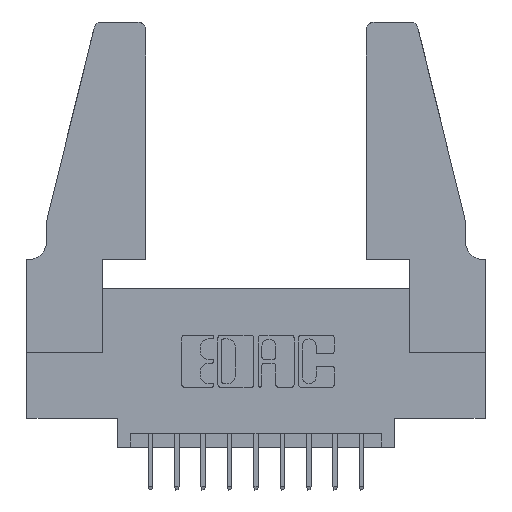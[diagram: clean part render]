
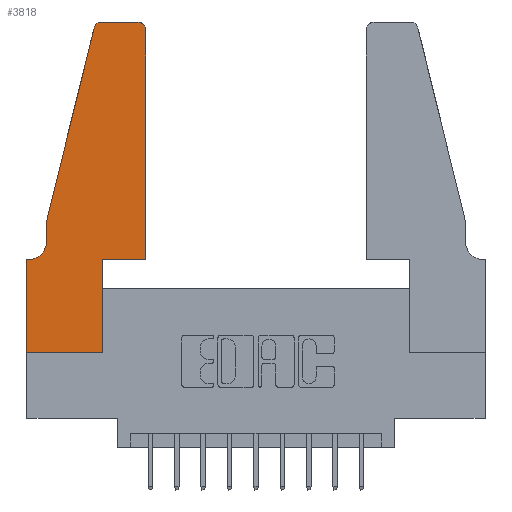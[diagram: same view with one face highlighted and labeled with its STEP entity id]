
A CAD part, top view. The second image highlights one B-rep face of the part: STEP entity #3818.
In plain terms, the highlighted planar face has unit normal (0, 0, 1).
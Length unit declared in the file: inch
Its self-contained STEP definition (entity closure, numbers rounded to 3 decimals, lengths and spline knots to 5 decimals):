
#101 = AXIS2_PLACEMENT_3D ( 'NONE', #13652, #8161, #7247 ) ;
#173 = CIRCLE ( 'NONE', #12254, 0.03 ) ;
#310 = CARTESIAN_POINT ( 'NONE',  ( 0.25487, 1.22718, 0.37 ) ) ;
#331 = DIRECTION ( 'NONE',  ( 0., 0., -1. ) ) ;
#516 = VECTOR ( 'NONE', #9417, 39.37008 ) ;
#571 = ORIENTED_EDGE ( 'NONE', *, *, #11517, .T. ) ;
#584 = DIRECTION ( 'NONE',  ( -0.239, -0.971, 0. ) ) ;
#972 = CARTESIAN_POINT ( 'NONE',  ( 0., 0., 0.37 ) ) ;
#1121 = LINE ( 'NONE', #11549, #13678 ) ;
#1203 = DIRECTION ( 'NONE',  ( 0., 0., 1. ) ) ;
#1227 = CARTESIAN_POINT ( 'NONE',  ( 0.2865, 0.35, 0.37 ) ) ;
#1270 = VERTEX_POINT ( 'NONE', #7177 ) ;
#1333 = ORIENTED_EDGE ( 'NONE', *, *, #12567, .T. ) ;
#2077 = CARTESIAN_POINT ( 'NONE',  ( 0.4505, 0.35, 0.37 ) ) ;
#2159 = ORIENTED_EDGE ( 'NONE', *, *, #5766, .T. ) ;
#2415 = VECTOR ( 'NONE', #11024, 39.37008 ) ;
#3048 = VERTEX_POINT ( 'NONE', #10202 ) ;
#3243 = CARTESIAN_POINT ( 'NONE',  ( 0.284, 1.25, 0.37 ) ) ;
#3503 = LINE ( 'NONE', #972, #10689 ) ;
#3506 = CARTESIAN_POINT ( 'NONE',  ( 0.0755, 0.42, 0.37 ) ) ;
#3565 = DIRECTION ( 'NONE',  ( -1., 0., 0. ) ) ;
#3571 = EDGE_LOOP ( 'NONE', ( #6645, #12556, #571, #2159, #7441, #1333, #13714, #7358, #8673, #13281, #11653, #7525 ) ) ;
#3768 = VERTEX_POINT ( 'NONE', #8648 ) ;
#3787 = VECTOR ( 'NONE', #7420, 39.37008 ) ;
#3810 = VECTOR ( 'NONE', #8436, 39.37008 ) ;
#3818 = ADVANCED_FACE ( 'NONE', ( #10408 ), #4012, .T. ) ;
#4012 = PLANE ( 'NONE',  #101 ) ;
#4269 = CARTESIAN_POINT ( 'NONE',  ( 0.4505, 0.35, 0.37 ) ) ;
#4739 = DIRECTION ( 'NONE',  ( 1., 0., 0. ) ) ;
#5197 = DIRECTION ( 'NONE',  ( 0., 1., 0. ) ) ;
#5241 = VERTEX_POINT ( 'NONE', #3243 ) ;
#5455 = CARTESIAN_POINT ( 'NONE',  ( 0.4505, 1.22, 0.37 ) ) ;
#5630 = CIRCLE ( 'NONE', #12448, 0.03 ) ;
#5703 = CARTESIAN_POINT ( 'NONE',  ( 0.284, 1.22, 0.37 ) ) ;
#5766 = EDGE_CURVE ( 'NONE', #6550, #9690, #7827, .T. ) ;
#5801 = CARTESIAN_POINT ( 'NONE',  ( 0.0755, 0.35, 0.37 ) ) ;
#5875 = VERTEX_POINT ( 'NONE', #4269 ) ;
#6411 = DIRECTION ( 'NONE',  ( 0., -1., 0. ) ) ;
#6478 = EDGE_CURVE ( 'NONE', #8548, #5875, #11326, .T. ) ;
#6481 = EDGE_CURVE ( 'NONE', #3048, #9802, #1121, .T. ) ;
#6500 = EDGE_CURVE ( 'NONE', #1270, #5241, #12181, .T. ) ;
#6550 = VERTEX_POINT ( 'NONE', #7520 ) ;
#6645 = ORIENTED_EDGE ( 'NONE', *, *, #6500, .T. ) ;
#7027 = EDGE_CURVE ( 'NONE', #9690, #3768, #12182, .T. ) ;
#7177 = CARTESIAN_POINT ( 'NONE',  ( 0.4205, 1.25, 0.37 ) ) ;
#7247 = DIRECTION ( 'NONE',  ( 1., 0., 0. ) ) ;
#7358 = ORIENTED_EDGE ( 'NONE', *, *, #9255, .T. ) ;
#7384 = LINE ( 'NONE', #11530, #516 ) ;
#7394 = CARTESIAN_POINT ( 'NONE',  ( 0.0755, 0.5, 0.37 ) ) ;
#7420 = DIRECTION ( 'NONE',  ( -1., 0., 0. ) ) ;
#7441 = ORIENTED_EDGE ( 'NONE', *, *, #7027, .T. ) ;
#7478 = VERTEX_POINT ( 'NONE', #9948 ) ;
#7520 = CARTESIAN_POINT ( 'NONE',  ( 0.0755, 0.5, 0.37 ) ) ;
#7525 = ORIENTED_EDGE ( 'NONE', *, *, #7656, .T. ) ;
#7656 = EDGE_CURVE ( 'NONE', #13601, #1270, #173, .T. ) ;
#7827 = LINE ( 'NONE', #7394, #3810 ) ;
#7829 = EDGE_CURVE ( 'NONE', #7478, #8548, #12726, .T. ) ;
#8161 = DIRECTION ( 'NONE',  ( 0., 0., 1. ) ) ;
#8436 = DIRECTION ( 'NONE',  ( 0., -1., 0. ) ) ;
#8548 = VERTEX_POINT ( 'NONE', #1227 ) ;
#8566 = CARTESIAN_POINT ( 'NONE',  ( 0.2605, 1.25, 0.37 ) ) ;
#8606 = LINE ( 'NONE', #5801, #2415 ) ;
#8629 = LINE ( 'NONE', #12074, #9614 ) ;
#8648 = CARTESIAN_POINT ( 'NONE',  ( 0.0055, 0.35, 0.37 ) ) ;
#8673 = ORIENTED_EDGE ( 'NONE', *, *, #7829, .T. ) ;
#8932 = CARTESIAN_POINT ( 'NONE',  ( 0.0055, 0.42, 0.37 ) ) ;
#9255 = EDGE_CURVE ( 'NONE', #9802, #7478, #3503, .T. ) ;
#9367 = VECTOR ( 'NONE', #5197, 39.37008 ) ;
#9417 = DIRECTION ( 'NONE',  ( 0., 1., 0. ) ) ;
#9614 = VECTOR ( 'NONE', #584, 39.37008 ) ;
#9690 = VERTEX_POINT ( 'NONE', #3506 ) ;
#9802 = VERTEX_POINT ( 'NONE', #13859 ) ;
#9948 = CARTESIAN_POINT ( 'NONE',  ( 0.2865, 0., 0.37 ) ) ;
#10202 = CARTESIAN_POINT ( 'NONE',  ( 0., 0.35, 0.37 ) ) ;
#10408 = FACE_OUTER_BOUND ( 'NONE', #3571, .T. ) ;
#10487 = VECTOR ( 'NONE', #10527, 39.37008 ) ;
#10527 = DIRECTION ( 'NONE',  ( 1., 0., 0. ) ) ;
#10567 = VERTEX_POINT ( 'NONE', #310 ) ;
#10689 = VECTOR ( 'NONE', #11695, 39.37008 ) ;
#11024 = DIRECTION ( 'NONE',  ( -1., 0., 0. ) ) ;
#11102 = EDGE_CURVE ( 'NONE', #5241, #10567, #5630, .T. ) ;
#11326 = LINE ( 'NONE', #2077, #10487 ) ;
#11517 = EDGE_CURVE ( 'NONE', #10567, #6550, #8629, .T. ) ;
#11530 = CARTESIAN_POINT ( 'NONE',  ( 0.4505, 0.35, 0.37 ) ) ;
#11549 = CARTESIAN_POINT ( 'NONE',  ( 0., 0., 0.37 ) ) ;
#11592 = CARTESIAN_POINT ( 'NONE',  ( 0.2865, 0.35, 0.37 ) ) ;
#11653 = ORIENTED_EDGE ( 'NONE', *, *, #13494, .T. ) ;
#11695 = DIRECTION ( 'NONE',  ( 1., 0., 0. ) ) ;
#11956 = CARTESIAN_POINT ( 'NONE',  ( 0.4205, 1.22, 0.37 ) ) ;
#12004 = DIRECTION ( 'NONE',  ( 0., 0., 1. ) ) ;
#12074 = CARTESIAN_POINT ( 'NONE',  ( 0.0755, 0.5, 0.37 ) ) ;
#12181 = LINE ( 'NONE', #8566, #3787 ) ;
#12182 = CIRCLE ( 'NONE', #13237, 0.07 ) ;
#12200 = DIRECTION ( 'NONE',  ( 1., 0., 0. ) ) ;
#12254 = AXIS2_PLACEMENT_3D ( 'NONE', #11956, #12004, #4739 ) ;
#12448 = AXIS2_PLACEMENT_3D ( 'NONE', #5703, #1203, #12200 ) ;
#12556 = ORIENTED_EDGE ( 'NONE', *, *, #11102, .T. ) ;
#12567 = EDGE_CURVE ( 'NONE', #3768, #3048, #8606, .T. ) ;
#12726 = LINE ( 'NONE', #11592, #9367 ) ;
#13237 = AXIS2_PLACEMENT_3D ( 'NONE', #8932, #331, #3565 ) ;
#13281 = ORIENTED_EDGE ( 'NONE', *, *, #6478, .T. ) ;
#13494 = EDGE_CURVE ( 'NONE', #5875, #13601, #7384, .T. ) ;
#13601 = VERTEX_POINT ( 'NONE', #5455 ) ;
#13652 = CARTESIAN_POINT ( 'NONE',  ( 0., 0.35, 0.37 ) ) ;
#13678 = VECTOR ( 'NONE', #6411, 39.37008 ) ;
#13714 = ORIENTED_EDGE ( 'NONE', *, *, #6481, .T. ) ;
#13859 = CARTESIAN_POINT ( 'NONE',  ( 0., 0., 0.37 ) ) ;
